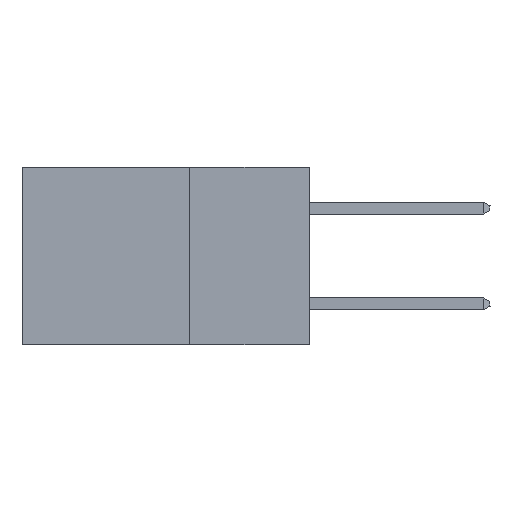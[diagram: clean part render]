
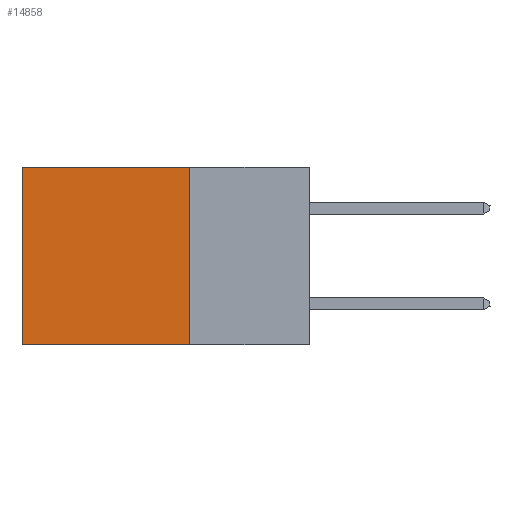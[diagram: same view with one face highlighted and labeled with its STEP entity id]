
A CAD part, left-side view. The second image highlights one B-rep face of the part: STEP entity #14858.
In plain terms, the highlighted planar face has unit normal (-1, 0, 0).
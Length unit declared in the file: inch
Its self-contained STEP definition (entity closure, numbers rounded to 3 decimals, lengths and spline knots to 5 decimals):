
#2149 = CARTESIAN_POINT ( 'NONE',  ( 0.2875, 0.25, 0. ) ) ;
#4830 = ORIENTED_EDGE ( 'NONE', *, *, #23205, .T. ) ;
#6102 = LINE ( 'NONE', #9248, #27268 ) ;
#6887 = VERTEX_POINT ( 'NONE', #18926 ) ;
#7055 = CARTESIAN_POINT ( 'NONE',  ( 0.2875, 0.25, 0. ) ) ;
#7498 = VERTEX_POINT ( 'NONE', #18650 ) ;
#9020 = CARTESIAN_POINT ( 'NONE',  ( 0.2875, 0.25, -0.37 ) ) ;
#9248 = CARTESIAN_POINT ( 'NONE',  ( 0.2875, 0.25, -0.37 ) ) ;
#9731 = DIRECTION ( 'NONE',  ( 0., 0., -1. ) ) ;
#9807 = ORIENTED_EDGE ( 'NONE', *, *, #30567, .F. ) ;
#12616 = DIRECTION ( 'NONE',  ( 1., 0., 0. ) ) ;
#12923 = ORIENTED_EDGE ( 'NONE', *, *, #14450, .F. ) ;
#13050 = CARTESIAN_POINT ( 'NONE',  ( 0.2875, 0.25, 0. ) ) ;
#14366 = VERTEX_POINT ( 'NONE', #13050 ) ;
#14450 = EDGE_CURVE ( 'NONE', #14366, #21387, #27203, .T. ) ;
#14858 = ADVANCED_FACE ( 'NONE', ( #18826 ), #22956, .F. ) ;
#17560 = DIRECTION ( 'NONE',  ( 0., 1., 0. ) ) ;
#18444 = VECTOR ( 'NONE', #20456, 39.37008 ) ;
#18650 = CARTESIAN_POINT ( 'NONE',  ( 0.2875, 0.6, -0.37 ) ) ;
#18773 = VECTOR ( 'NONE', #31333, 39.37008 ) ;
#18826 = FACE_OUTER_BOUND ( 'NONE', #25184, .T. ) ;
#18926 = CARTESIAN_POINT ( 'NONE',  ( 0.2875, 0.6, 0. ) ) ;
#19942 = DIRECTION ( 'NONE',  ( 0., 0., -1. ) ) ;
#20284 = ORIENTED_EDGE ( 'NONE', *, *, #23451, .T. ) ;
#20456 = DIRECTION ( 'NONE',  ( 0., 0., -1. ) ) ;
#21387 = VERTEX_POINT ( 'NONE', #9020 ) ;
#22956 = PLANE ( 'NONE',  #30200 ) ;
#23205 = EDGE_CURVE ( 'NONE', #14366, #6887, #26684, .T. ) ;
#23451 = EDGE_CURVE ( 'NONE', #6887, #7498, #27913, .T. ) ;
#25184 = EDGE_LOOP ( 'NONE', ( #20284, #9807, #12923, #4830 ) ) ;
#25293 = CARTESIAN_POINT ( 'NONE',  ( 0.2875, 0.6, 0. ) ) ;
#26684 = LINE ( 'NONE', #28804, #18773 ) ;
#27203 = LINE ( 'NONE', #2149, #18444 ) ;
#27268 = VECTOR ( 'NONE', #17560, 39.37008 ) ;
#27913 = LINE ( 'NONE', #25293, #28758 ) ;
#28758 = VECTOR ( 'NONE', #19942, 39.37008 ) ;
#28804 = CARTESIAN_POINT ( 'NONE',  ( 0.2875, 0.25, 0. ) ) ;
#30200 = AXIS2_PLACEMENT_3D ( 'NONE', #7055, #12616, #9731 ) ;
#30567 = EDGE_CURVE ( 'NONE', #21387, #7498, #6102, .T. ) ;
#31333 = DIRECTION ( 'NONE',  ( 0., 1., 0. ) ) ;
